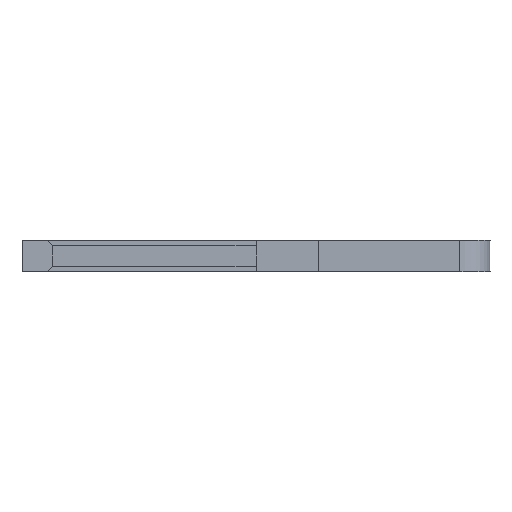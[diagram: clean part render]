
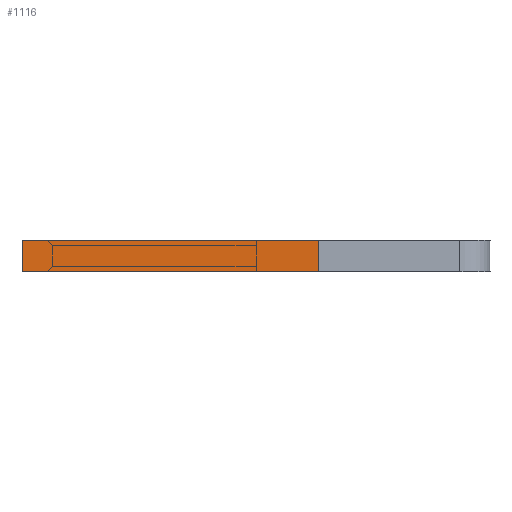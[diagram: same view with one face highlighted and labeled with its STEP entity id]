
A CAD part, left-side view. The second image highlights one B-rep face of the part: STEP entity #1116.
In plain terms, the highlighted face is planar.
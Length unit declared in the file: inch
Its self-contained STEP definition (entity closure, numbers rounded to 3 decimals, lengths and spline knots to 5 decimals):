
#147 = ORIENTED_EDGE ( 'NONE', *, *, #1612, .F. ) ;
#152 = VERTEX_POINT ( 'NONE', #2311 ) ;
#226 = EDGE_CURVE ( 'NONE', #809, #920, #1749, .T. ) ;
#234 = AXIS2_PLACEMENT_3D ( 'NONE', #534, #360, #1454 ) ;
#342 = CARTESIAN_POINT ( 'NONE',  ( 0.01, 0.15, -0.04 ) ) ;
#360 = DIRECTION ( 'NONE',  ( 0., 0., 1. ) ) ;
#470 = EDGE_CURVE ( 'NONE', #152, #624, #1465, .T. ) ;
#534 = CARTESIAN_POINT ( 'NONE',  ( 0.01, 0.15, -0.04 ) ) ;
#548 = EDGE_LOOP ( 'NONE', ( #922, #1702, #147, #1960 ) ) ;
#584 = DIRECTION ( 'NONE',  ( 0., 1., 0. ) ) ;
#624 = VERTEX_POINT ( 'NONE', #1407 ) ;
#723 = PLANE ( 'NONE',  #234 ) ;
#809 = VERTEX_POINT ( 'NONE', #342 ) ;
#920 = VERTEX_POINT ( 'NONE', #1259 ) ;
#922 = ORIENTED_EDGE ( 'NONE', *, *, #1886, .T. ) ;
#976 = VECTOR ( 'NONE', #2144, 39.37008 ) ;
#1006 = CARTESIAN_POINT ( 'NONE',  ( -0.01, 0.15, -0.04 ) ) ;
#1116 = ADVANCED_FACE ( 'NONE', ( #1923 ), #723, .F. ) ;
#1259 = CARTESIAN_POINT ( 'NONE',  ( -0.01, 0.15, -0.04 ) ) ;
#1299 = VECTOR ( 'NONE', #584, 39.37008 ) ;
#1371 = VECTOR ( 'NONE', #2318, 39.37008 ) ;
#1407 = CARTESIAN_POINT ( 'NONE',  ( -0.01, -0.04, -0.04 ) ) ;
#1454 = DIRECTION ( 'NONE',  ( 1., 0., 0. ) ) ;
#1465 = LINE ( 'NONE', #2290, #976 ) ;
#1612 = EDGE_CURVE ( 'NONE', #152, #809, #2292, .T. ) ;
#1669 = CARTESIAN_POINT ( 'NONE',  ( 0.01, 0.15, -0.04 ) ) ;
#1702 = ORIENTED_EDGE ( 'NONE', *, *, #226, .F. ) ;
#1749 = LINE ( 'NONE', #2113, #1371 ) ;
#1886 = EDGE_CURVE ( 'NONE', #624, #920, #2002, .T. ) ;
#1923 = FACE_OUTER_BOUND ( 'NONE', #548, .T. ) ;
#1960 = ORIENTED_EDGE ( 'NONE', *, *, #470, .T. ) ;
#2002 = LINE ( 'NONE', #1006, #2032 ) ;
#2032 = VECTOR ( 'NONE', #2082, 39.37008 ) ;
#2082 = DIRECTION ( 'NONE',  ( 0., 1., 0. ) ) ;
#2113 = CARTESIAN_POINT ( 'NONE',  ( 0.01, 0.15, -0.04 ) ) ;
#2144 = DIRECTION ( 'NONE',  ( -1., 0., 0. ) ) ;
#2290 = CARTESIAN_POINT ( 'NONE',  ( 0.01, -0.04, -0.04 ) ) ;
#2292 = LINE ( 'NONE', #1669, #1299 ) ;
#2311 = CARTESIAN_POINT ( 'NONE',  ( 0.01, -0.04, -0.04 ) ) ;
#2318 = DIRECTION ( 'NONE',  ( -1., 0., 0. ) ) ;
